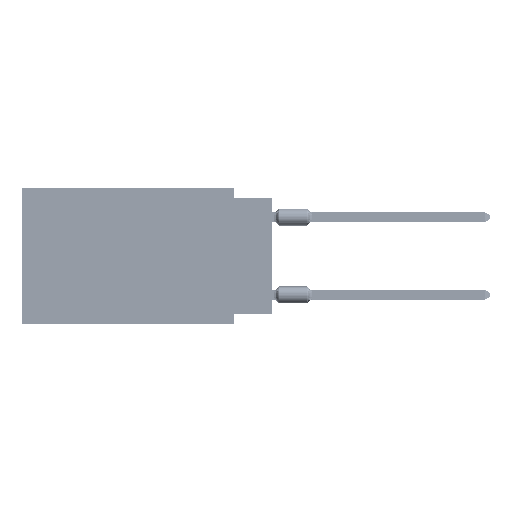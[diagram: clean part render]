
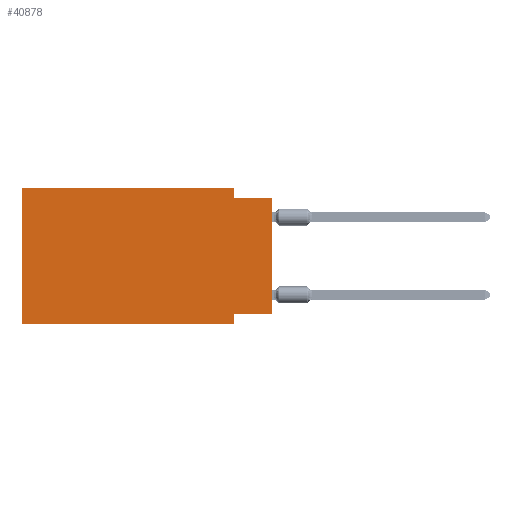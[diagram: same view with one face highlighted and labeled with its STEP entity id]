
A CAD part, left-side view. The second image highlights one B-rep face of the part: STEP entity #40878.
In plain terms, the highlighted planar face has unit normal (-1, 0, 0).
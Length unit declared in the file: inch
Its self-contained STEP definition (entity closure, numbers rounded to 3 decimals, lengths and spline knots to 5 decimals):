
#1836 = VERTEX_POINT ( 'NONE', #64510 ) ;
#7473 = VERTEX_POINT ( 'NONE', #20927 ) ;
#7859 = DIRECTION ( 'NONE',  ( 0., 0., 1. ) ) ;
#8588 = CARTESIAN_POINT ( 'NONE',  ( 0., 0.1, -0.35 ) ) ;
#10908 = CARTESIAN_POINT ( 'NONE',  ( 0., 0.645, -0.35 ) ) ;
#14160 = LINE ( 'NONE', #80040, #28853 ) ;
#14690 = VERTEX_POINT ( 'NONE', #121311 ) ;
#18888 = LINE ( 'NONE', #10908, #92907 ) ;
#18976 = EDGE_CURVE ( 'NONE', #108905, #61495, #18888, .T. ) ;
#19598 = CARTESIAN_POINT ( 'NONE',  ( 0., 0.1, 0. ) ) ;
#20927 = CARTESIAN_POINT ( 'NONE',  ( 0., 0.1, -0.025 ) ) ;
#25182 = VECTOR ( 'NONE', #7859, 39.37008 ) ;
#26837 = EDGE_CURVE ( 'NONE', #88802, #14690, #38003, .T. ) ;
#28296 = EDGE_CURVE ( 'NONE', #108905, #55003, #95543, .T. ) ;
#28853 = VECTOR ( 'NONE', #71435, 39.37008 ) ;
#32779 = EDGE_CURVE ( 'NONE', #88802, #88265, #57946, .T. ) ;
#32812 = LINE ( 'NONE', #50672, #77956 ) ;
#33568 = EDGE_LOOP ( 'NONE', ( #101960, #117843, #71079, #114856, #41953, #69071, #58225, #94099 ) ) ;
#36533 = EDGE_CURVE ( 'NONE', #88265, #61495, #55354, .T. ) ;
#38003 = LINE ( 'NONE', #76180, #25182 ) ;
#38230 = CARTESIAN_POINT ( 'NONE',  ( 0., 0., -0.325 ) ) ;
#39913 = DIRECTION ( 'NONE',  ( 0., 0., -1. ) ) ;
#40878 = ADVANCED_FACE ( 'NONE', ( #51704 ), #42462, .F. ) ;
#41953 = ORIENTED_EDGE ( 'NONE', *, *, #28296, .F. ) ;
#42462 = PLANE ( 'NONE',  #50629 ) ;
#48664 = DIRECTION ( 'NONE',  ( 0., 1., 0. ) ) ;
#50629 = AXIS2_PLACEMENT_3D ( 'NONE', #97312, #78818, #89296 ) ;
#50672 = CARTESIAN_POINT ( 'NONE',  ( 0., 0., -0.025 ) ) ;
#51704 = FACE_OUTER_BOUND ( 'NONE', #33568, .T. ) ;
#51883 = CARTESIAN_POINT ( 'NONE',  ( 0., 0.645, 0. ) ) ;
#55003 = VERTEX_POINT ( 'NONE', #51883 ) ;
#55354 = LINE ( 'NONE', #8588, #94156 ) ;
#56140 = EDGE_CURVE ( 'NONE', #7473, #14690, #32812, .T. ) ;
#57946 = LINE ( 'NONE', #38230, #85465 ) ;
#58225 = ORIENTED_EDGE ( 'NONE', *, *, #36533, .F. ) ;
#61147 = DIRECTION ( 'NONE',  ( 0., -1., 0. ) ) ;
#61495 = VERTEX_POINT ( 'NONE', #85654 ) ;
#63122 = EDGE_CURVE ( 'NONE', #1836, #7473, #95380, .T. ) ;
#64510 = CARTESIAN_POINT ( 'NONE',  ( 0., 0.1, 0. ) ) ;
#69071 = ORIENTED_EDGE ( 'NONE', *, *, #18976, .T. ) ;
#71079 = ORIENTED_EDGE ( 'NONE', *, *, #63122, .F. ) ;
#71435 = DIRECTION ( 'NONE',  ( 0., -1., 0. ) ) ;
#72331 = CARTESIAN_POINT ( 'NONE',  ( 0., 0.1, -0.325 ) ) ;
#74055 = CARTESIAN_POINT ( 'NONE',  ( 0., 0.645, -0.35 ) ) ;
#76180 = CARTESIAN_POINT ( 'NONE',  ( 0., 0., 0. ) ) ;
#77956 = VECTOR ( 'NONE', #61147, 39.37008 ) ;
#78818 = DIRECTION ( 'NONE',  ( 1., 0., 0. ) ) ;
#80040 = CARTESIAN_POINT ( 'NONE',  ( 0., 0.645, 0. ) ) ;
#85465 = VECTOR ( 'NONE', #48664, 39.37008 ) ;
#85654 = CARTESIAN_POINT ( 'NONE',  ( 0., 0.1, -0.35 ) ) ;
#88265 = VERTEX_POINT ( 'NONE', #72331 ) ;
#88802 = VERTEX_POINT ( 'NONE', #94924 ) ;
#89296 = DIRECTION ( 'NONE',  ( 0., 0., -1. ) ) ;
#92247 = VECTOR ( 'NONE', #103555, 39.37008 ) ;
#92907 = VECTOR ( 'NONE', #97669, 39.37008 ) ;
#92950 = DIRECTION ( 'NONE',  ( 0., 0., -1. ) ) ;
#94099 = ORIENTED_EDGE ( 'NONE', *, *, #32779, .F. ) ;
#94156 = VECTOR ( 'NONE', #92950, 39.37008 ) ;
#94924 = CARTESIAN_POINT ( 'NONE',  ( 0., 0., -0.325 ) ) ;
#95380 = LINE ( 'NONE', #19598, #120077 ) ;
#95543 = LINE ( 'NONE', #111577, #92247 ) ;
#97312 = CARTESIAN_POINT ( 'NONE',  ( 0., 0.645, 0. ) ) ;
#97669 = DIRECTION ( 'NONE',  ( 0., -1., 0. ) ) ;
#99044 = EDGE_CURVE ( 'NONE', #55003, #1836, #14160, .T. ) ;
#101960 = ORIENTED_EDGE ( 'NONE', *, *, #26837, .T. ) ;
#103555 = DIRECTION ( 'NONE',  ( 0., 0., 1. ) ) ;
#108905 = VERTEX_POINT ( 'NONE', #74055 ) ;
#111577 = CARTESIAN_POINT ( 'NONE',  ( 0., 0.645, 0. ) ) ;
#114856 = ORIENTED_EDGE ( 'NONE', *, *, #99044, .F. ) ;
#117843 = ORIENTED_EDGE ( 'NONE', *, *, #56140, .F. ) ;
#120077 = VECTOR ( 'NONE', #39913, 39.37008 ) ;
#121311 = CARTESIAN_POINT ( 'NONE',  ( 0., 0., -0.025 ) ) ;
